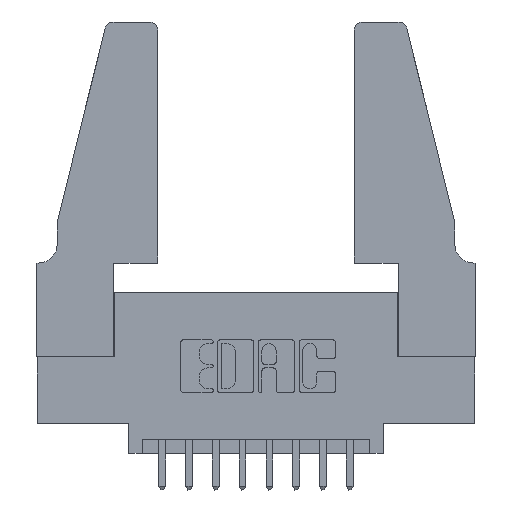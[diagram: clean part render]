
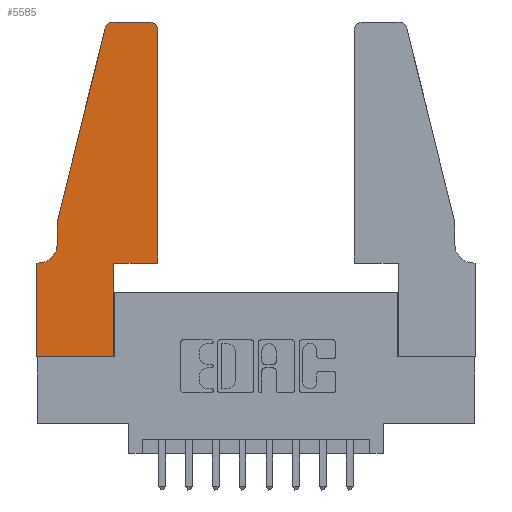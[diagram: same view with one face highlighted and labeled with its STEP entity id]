
A CAD part, top view. The second image highlights one B-rep face of the part: STEP entity #5585.
In plain terms, the highlighted planar face has unit normal (0, 0, 1).
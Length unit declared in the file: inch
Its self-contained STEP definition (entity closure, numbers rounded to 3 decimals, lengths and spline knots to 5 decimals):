
#223 = EDGE_CURVE ( 'NONE', #8662, #13082, #3391, .T. ) ;
#366 = ORIENTED_EDGE ( 'NONE', *, *, #2898, .T. ) ;
#835 = EDGE_CURVE ( 'NONE', #3238, #1592, #6881, .T. ) ;
#1068 = DIRECTION ( 'NONE',  ( 0., 0., 1. ) ) ;
#1147 = ORIENTED_EDGE ( 'NONE', *, *, #835, .T. ) ;
#1347 = CARTESIAN_POINT ( 'NONE',  ( 0., 0.35, 0.37 ) ) ;
#1358 = DIRECTION ( 'NONE',  ( -1., 0., 0. ) ) ;
#1389 = VECTOR ( 'NONE', #7162, 39.37008 ) ;
#1461 = CARTESIAN_POINT ( 'NONE',  ( 0.4205, 1.22, 0.37 ) ) ;
#1592 = VERTEX_POINT ( 'NONE', #8911 ) ;
#2036 = VECTOR ( 'NONE', #9429, 39.37008 ) ;
#2243 = CIRCLE ( 'NONE', #7086, 0.07 ) ;
#2262 = EDGE_CURVE ( 'NONE', #8753, #12715, #4335, .T. ) ;
#2293 = FACE_OUTER_BOUND ( 'NONE', #10489, .T. ) ;
#2366 = LINE ( 'NONE', #10886, #2036 ) ;
#2416 = CARTESIAN_POINT ( 'NONE',  ( 0.2605, 1.25, 0.37 ) ) ;
#2480 = VECTOR ( 'NONE', #6199, 39.37008 ) ;
#2542 = DIRECTION ( 'NONE',  ( 1., 0., 0. ) ) ;
#2562 = AXIS2_PLACEMENT_3D ( 'NONE', #1461, #8599, #2542 ) ;
#2582 = CIRCLE ( 'NONE', #2562, 0.03 ) ;
#2812 = LINE ( 'NONE', #4352, #7879 ) ;
#2898 = EDGE_CURVE ( 'NONE', #5357, #8753, #2366, .T. ) ;
#3110 = VECTOR ( 'NONE', #6525, 39.37008 ) ;
#3224 = CARTESIAN_POINT ( 'NONE',  ( 0., 0.35, 0.37 ) ) ;
#3238 = VERTEX_POINT ( 'NONE', #6388 ) ;
#3365 = CARTESIAN_POINT ( 'NONE',  ( 0., 0., 0.37 ) ) ;
#3391 = LINE ( 'NONE', #9687, #5470 ) ;
#3411 = CARTESIAN_POINT ( 'NONE',  ( 0.4205, 1.25, 0.37 ) ) ;
#3432 = EDGE_CURVE ( 'NONE', #13082, #12362, #9178, .T. ) ;
#4144 = VECTOR ( 'NONE', #11961, 39.37008 ) ;
#4265 = PLANE ( 'NONE',  #10882 ) ;
#4335 = LINE ( 'NONE', #3365, #7019 ) ;
#4341 = DIRECTION ( 'NONE',  ( 0., 0., -1. ) ) ;
#4352 = CARTESIAN_POINT ( 'NONE',  ( 0., 0., 0.37 ) ) ;
#4716 = CARTESIAN_POINT ( 'NONE',  ( 0.284, 1.25, 0.37 ) ) ;
#4733 = CARTESIAN_POINT ( 'NONE',  ( 0., 0., 0.37 ) ) ;
#4858 = EDGE_CURVE ( 'NONE', #5972, #8662, #5221, .T. ) ;
#5092 = VERTEX_POINT ( 'NONE', #3411 ) ;
#5178 = ORIENTED_EDGE ( 'NONE', *, *, #4858, .T. ) ;
#5188 = CARTESIAN_POINT ( 'NONE',  ( 0.4505, 0.35, 0.37 ) ) ;
#5221 = LINE ( 'NONE', #9158, #2480 ) ;
#5283 = DIRECTION ( 'NONE',  ( 0., 0., 1. ) ) ;
#5357 = VERTEX_POINT ( 'NONE', #12887 ) ;
#5470 = VECTOR ( 'NONE', #10707, 39.37008 ) ;
#5581 = ORIENTED_EDGE ( 'NONE', *, *, #12621, .T. ) ;
#5585 = ADVANCED_FACE ( 'NONE', ( #2293 ), #4265, .T. ) ;
#5688 = ORIENTED_EDGE ( 'NONE', *, *, #10620, .T. ) ;
#5728 = EDGE_CURVE ( 'NONE', #1592, #8210, #11119, .T. ) ;
#5972 = VERTEX_POINT ( 'NONE', #8954 ) ;
#6138 = CARTESIAN_POINT ( 'NONE',  ( 0.4505, 1.22, 0.37 ) ) ;
#6199 = DIRECTION ( 'NONE',  ( 0., 1., 0. ) ) ;
#6388 = CARTESIAN_POINT ( 'NONE',  ( 0.25487, 1.22718, 0.37 ) ) ;
#6525 = DIRECTION ( 'NONE',  ( 0., -1., 0. ) ) ;
#6542 = CARTESIAN_POINT ( 'NONE',  ( 0.0755, 0.42, 0.37 ) ) ;
#6881 = LINE ( 'NONE', #11234, #1389 ) ;
#7019 = VECTOR ( 'NONE', #10983, 39.37008 ) ;
#7060 = ORIENTED_EDGE ( 'NONE', *, *, #7368, .T. ) ;
#7086 = AXIS2_PLACEMENT_3D ( 'NONE', #10331, #4341, #11319 ) ;
#7162 = DIRECTION ( 'NONE',  ( -0.239, -0.971, 0. ) ) ;
#7209 = CARTESIAN_POINT ( 'NONE',  ( 0.284, 1.22, 0.37 ) ) ;
#7368 = EDGE_CURVE ( 'NONE', #7689, #3238, #10787, .T. ) ;
#7689 = VERTEX_POINT ( 'NONE', #4716 ) ;
#7879 = VECTOR ( 'NONE', #10345, 39.37008 ) ;
#8147 = VECTOR ( 'NONE', #1358, 39.37008 ) ;
#8210 = VERTEX_POINT ( 'NONE', #6542 ) ;
#8212 = DIRECTION ( 'NONE',  ( 1., 0., 0. ) ) ;
#8599 = DIRECTION ( 'NONE',  ( 0., 0., 1. ) ) ;
#8662 = VERTEX_POINT ( 'NONE', #9402 ) ;
#8753 = VERTEX_POINT ( 'NONE', #1347 ) ;
#8911 = CARTESIAN_POINT ( 'NONE',  ( 0.0755, 0.5, 0.37 ) ) ;
#8954 = CARTESIAN_POINT ( 'NONE',  ( 0.2865, 0., 0.37 ) ) ;
#9158 = CARTESIAN_POINT ( 'NONE',  ( 0.2865, 0.35, 0.37 ) ) ;
#9178 = LINE ( 'NONE', #11308, #4144 ) ;
#9402 = CARTESIAN_POINT ( 'NONE',  ( 0.2865, 0.35, 0.37 ) ) ;
#9429 = DIRECTION ( 'NONE',  ( -1., 0., 0. ) ) ;
#9687 = CARTESIAN_POINT ( 'NONE',  ( 0.4505, 0.35, 0.37 ) ) ;
#10037 = ORIENTED_EDGE ( 'NONE', *, *, #5728, .T. ) ;
#10331 = CARTESIAN_POINT ( 'NONE',  ( 0.0055, 0.42, 0.37 ) ) ;
#10345 = DIRECTION ( 'NONE',  ( 1., 0., 0. ) ) ;
#10455 = CARTESIAN_POINT ( 'NONE',  ( 0.0755, 0.5, 0.37 ) ) ;
#10489 = EDGE_LOOP ( 'NONE', ( #10965, #7060, #1147, #10037, #10494, #366, #12136, #5688, #5178, #12814, #10911, #5581 ) ) ;
#10494 = ORIENTED_EDGE ( 'NONE', *, *, #13140, .T. ) ;
#10620 = EDGE_CURVE ( 'NONE', #12715, #5972, #2812, .T. ) ;
#10707 = DIRECTION ( 'NONE',  ( 1., 0., 0. ) ) ;
#10787 = CIRCLE ( 'NONE', #12452, 0.03 ) ;
#10794 = LINE ( 'NONE', #2416, #8147 ) ;
#10882 = AXIS2_PLACEMENT_3D ( 'NONE', #3224, #5283, #12245 ) ;
#10886 = CARTESIAN_POINT ( 'NONE',  ( 0.0755, 0.35, 0.37 ) ) ;
#10911 = ORIENTED_EDGE ( 'NONE', *, *, #3432, .T. ) ;
#10965 = ORIENTED_EDGE ( 'NONE', *, *, #11872, .T. ) ;
#10983 = DIRECTION ( 'NONE',  ( 0., -1., 0. ) ) ;
#11119 = LINE ( 'NONE', #10455, #3110 ) ;
#11234 = CARTESIAN_POINT ( 'NONE',  ( 0.0755, 0.5, 0.37 ) ) ;
#11308 = CARTESIAN_POINT ( 'NONE',  ( 0.4505, 0.35, 0.37 ) ) ;
#11319 = DIRECTION ( 'NONE',  ( -1., 0., 0. ) ) ;
#11872 = EDGE_CURVE ( 'NONE', #5092, #7689, #10794, .T. ) ;
#11961 = DIRECTION ( 'NONE',  ( 0., 1., 0. ) ) ;
#12136 = ORIENTED_EDGE ( 'NONE', *, *, #2262, .T. ) ;
#12245 = DIRECTION ( 'NONE',  ( 1., 0., 0. ) ) ;
#12362 = VERTEX_POINT ( 'NONE', #6138 ) ;
#12452 = AXIS2_PLACEMENT_3D ( 'NONE', #7209, #1068, #8212 ) ;
#12621 = EDGE_CURVE ( 'NONE', #12362, #5092, #2582, .T. ) ;
#12715 = VERTEX_POINT ( 'NONE', #4733 ) ;
#12814 = ORIENTED_EDGE ( 'NONE', *, *, #223, .T. ) ;
#12887 = CARTESIAN_POINT ( 'NONE',  ( 0.0055, 0.35, 0.37 ) ) ;
#13082 = VERTEX_POINT ( 'NONE', #5188 ) ;
#13140 = EDGE_CURVE ( 'NONE', #8210, #5357, #2243, .T. ) ;
